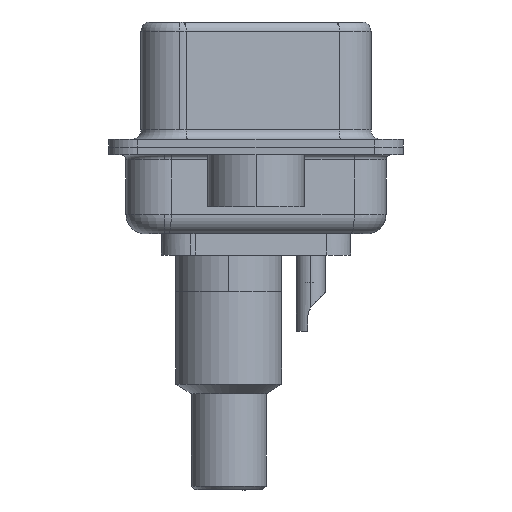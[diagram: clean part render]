
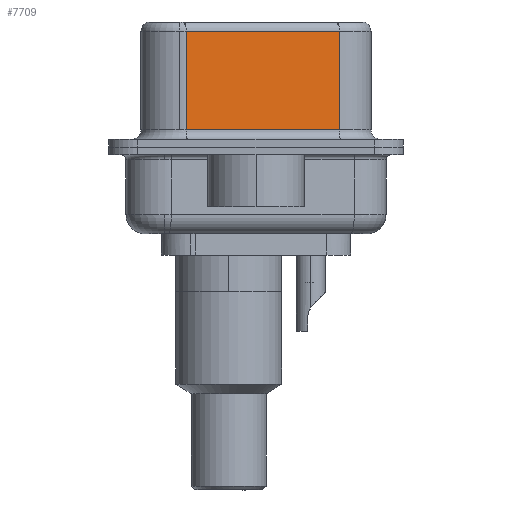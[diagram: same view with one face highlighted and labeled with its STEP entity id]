
A CAD part, left-side view. The second image highlights one B-rep face of the part: STEP entity #7709.
In plain terms, the highlighted planar face has unit normal (-0.985, -0.174, 0).
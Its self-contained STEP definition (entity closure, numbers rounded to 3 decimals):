
#1226 = CARTESIAN_POINT ( 'NONE',  ( 5.132, -4.322, 6.52 ) ) ;
#2826 = CARTESIAN_POINT ( 'NONE',  ( 5.132, -4.322, 0.9 ) ) ;
#5073 = VECTOR ( 'NONE', #7497, 1000. ) ;
#5189 = CARTESIAN_POINT ( 'NONE',  ( 5.132, -4.322, 6.02 ) ) ;
#6595 = VERTEX_POINT ( 'NONE', #13523 ) ;
#7497 = DIRECTION ( 'NONE',  ( 0.174, -0.985, 0. ) ) ;
#7709 = ADVANCED_FACE ( 'NONE', ( #29229 ), #29566, .F. ) ;
#8503 = VECTOR ( 'NONE', #17427, 1000. ) ;
#9231 = LINE ( 'NONE', #1226, #8503 ) ;
#9391 = EDGE_CURVE ( 'NONE', #20934, #19581, #9231, .T. ) ;
#9685 = CARTESIAN_POINT ( 'NONE',  ( 3.73, 3.628, 6.02 ) ) ;
#11572 = VECTOR ( 'NONE', #12127, 1000. ) ;
#11586 = ORIENTED_EDGE ( 'NONE', *, *, #9391, .F. ) ;
#12127 = DIRECTION ( 'NONE',  ( -0.174, 0.985, 0. ) ) ;
#12425 = ORIENTED_EDGE ( 'NONE', *, *, #20244, .T. ) ;
#13131 = CARTESIAN_POINT ( 'NONE',  ( 3.73, 3.628, 6.52 ) ) ;
#13523 = CARTESIAN_POINT ( 'NONE',  ( 3.73, 3.628, 0.9 ) ) ;
#14410 = CARTESIAN_POINT ( 'NONE',  ( 5.132, -4.322, 6.02 ) ) ;
#14913 = LINE ( 'NONE', #13131, #26519 ) ;
#15651 = VERTEX_POINT ( 'NONE', #9685 ) ;
#17327 = LINE ( 'NONE', #2826, #5073 ) ;
#17427 = DIRECTION ( 'NONE',  ( 0., 0., -1. ) ) ;
#17526 = EDGE_LOOP ( 'NONE', ( #11586, #12425, #29134, #18618 ) ) ;
#17683 = LINE ( 'NONE', #5189, #11572 ) ;
#18618 = ORIENTED_EDGE ( 'NONE', *, *, #22751, .T. ) ;
#19581 = VERTEX_POINT ( 'NONE', #25541 ) ;
#20244 = EDGE_CURVE ( 'NONE', #20934, #15651, #17683, .T. ) ;
#20934 = VERTEX_POINT ( 'NONE', #14410 ) ;
#22751 = EDGE_CURVE ( 'NONE', #6595, #19581, #17327, .T. ) ;
#25541 = CARTESIAN_POINT ( 'NONE',  ( 5.132, -4.322, 0.9 ) ) ;
#26519 = VECTOR ( 'NONE', #29459, 1000. ) ;
#26602 = AXIS2_PLACEMENT_3D ( 'NONE', #28359, #27944, #27845 ) ;
#27092 = EDGE_CURVE ( 'NONE', #15651, #6595, #14913, .T. ) ;
#27845 = DIRECTION ( 'NONE',  ( -0.174, 0.985, 0. ) ) ;
#27944 = DIRECTION ( 'NONE',  ( 0.985, 0.174, 0. ) ) ;
#28359 = CARTESIAN_POINT ( 'NONE',  ( 5.132, -4.322, 6.52 ) ) ;
#29134 = ORIENTED_EDGE ( 'NONE', *, *, #27092, .T. ) ;
#29229 = FACE_OUTER_BOUND ( 'NONE', #17526, .T. ) ;
#29459 = DIRECTION ( 'NONE',  ( 0., 0., -1. ) ) ;
#29566 = PLANE ( 'NONE',  #26602 ) ;
